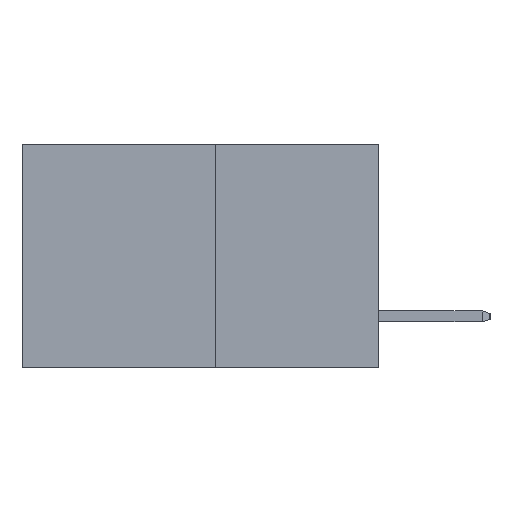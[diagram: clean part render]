
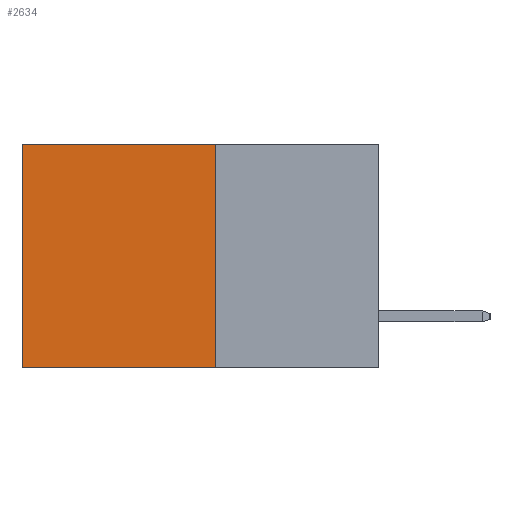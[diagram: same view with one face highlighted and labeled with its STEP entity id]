
A CAD part, left-side view. The second image highlights one B-rep face of the part: STEP entity #2634.
In plain terms, the highlighted planar face has unit normal (-1, 0, 0).
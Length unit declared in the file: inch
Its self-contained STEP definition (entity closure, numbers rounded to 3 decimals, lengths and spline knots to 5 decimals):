
#185 = DIRECTION ( 'NONE',  ( 1., 0., 0. ) ) ;
#229 = VERTEX_POINT ( 'NONE', #8804 ) ;
#544 = ORIENTED_EDGE ( 'NONE', *, *, #2525, .T. ) ;
#1174 = CARTESIAN_POINT ( 'NONE',  ( 0.277, 0.27, -0.37 ) ) ;
#1684 = CARTESIAN_POINT ( 'NONE',  ( 0.277, 0.27, 0. ) ) ;
#2006 = DIRECTION ( 'NONE',  ( 0., 0., -1. ) ) ;
#2490 = LINE ( 'NONE', #9467, #4247 ) ;
#2525 = EDGE_CURVE ( 'NONE', #7973, #3474, #2490, .T. ) ;
#2634 = ADVANCED_FACE ( 'NONE', ( #7252 ), #8473, .F. ) ;
#2893 = LINE ( 'NONE', #1684, #7915 ) ;
#2967 = CARTESIAN_POINT ( 'NONE',  ( 0.277, 0.27, -0.37 ) ) ;
#2987 = VECTOR ( 'NONE', #9592, 39.37008 ) ;
#3447 = LINE ( 'NONE', #1174, #2987 ) ;
#3474 = VERTEX_POINT ( 'NONE', #7965 ) ;
#3509 = DIRECTION ( 'NONE',  ( 0., 0., -1. ) ) ;
#3660 = DIRECTION ( 'NONE',  ( 0., 1., 0. ) ) ;
#3924 = AXIS2_PLACEMENT_3D ( 'NONE', #4415, #185, #3509 ) ;
#4247 = VECTOR ( 'NONE', #2006, 39.37008 ) ;
#4324 = VECTOR ( 'NONE', #4425, 39.37008 ) ;
#4415 = CARTESIAN_POINT ( 'NONE',  ( 0.277, 0.27, -0.37 ) ) ;
#4425 = DIRECTION ( 'NONE',  ( 0., 0., -1. ) ) ;
#4548 = LINE ( 'NONE', #2967, #4324 ) ;
#5020 = ORIENTED_EDGE ( 'NONE', *, *, #7574, .F. ) ;
#5464 = ORIENTED_EDGE ( 'NONE', *, *, #7235, .T. ) ;
#5613 = EDGE_LOOP ( 'NONE', ( #544, #5020, #7047, #5464 ) ) ;
#5767 = CARTESIAN_POINT ( 'NONE',  ( 0.277, 0.27, 0. ) ) ;
#7047 = ORIENTED_EDGE ( 'NONE', *, *, #9123, .F. ) ;
#7235 = EDGE_CURVE ( 'NONE', #7330, #7973, #2893, .T. ) ;
#7252 = FACE_OUTER_BOUND ( 'NONE', #5613, .T. ) ;
#7330 = VERTEX_POINT ( 'NONE', #5767 ) ;
#7574 = EDGE_CURVE ( 'NONE', #229, #3474, #3447, .T. ) ;
#7915 = VECTOR ( 'NONE', #3660, 39.37008 ) ;
#7965 = CARTESIAN_POINT ( 'NONE',  ( 0.277, 0.59, -0.37 ) ) ;
#7973 = VERTEX_POINT ( 'NONE', #9341 ) ;
#8473 = PLANE ( 'NONE',  #3924 ) ;
#8804 = CARTESIAN_POINT ( 'NONE',  ( 0.277, 0.27, -0.37 ) ) ;
#9123 = EDGE_CURVE ( 'NONE', #7330, #229, #4548, .T. ) ;
#9341 = CARTESIAN_POINT ( 'NONE',  ( 0.277, 0.59, 0. ) ) ;
#9467 = CARTESIAN_POINT ( 'NONE',  ( 0.277, 0.59, -0.37 ) ) ;
#9592 = DIRECTION ( 'NONE',  ( 0., 1., 0. ) ) ;
